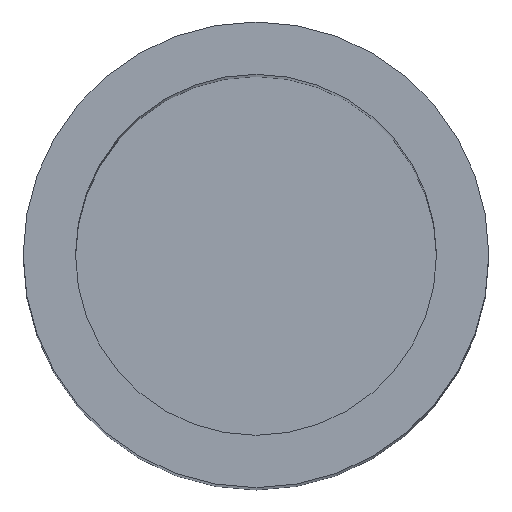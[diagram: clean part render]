
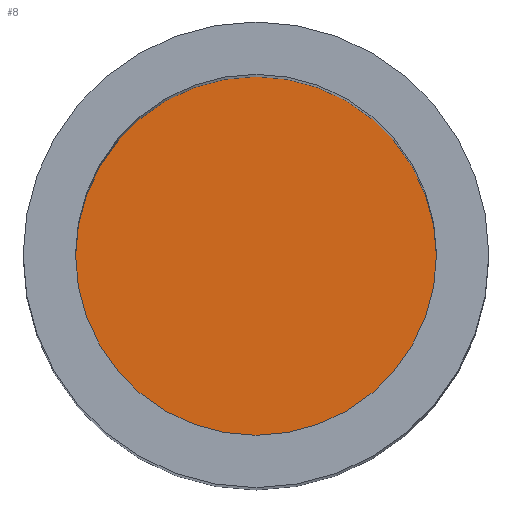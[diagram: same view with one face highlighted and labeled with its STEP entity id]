
A CAD part, top view. The second image highlights one B-rep face of the part: STEP entity #8.
In plain terms, the highlighted planar face has unit normal (0, 0, 1).
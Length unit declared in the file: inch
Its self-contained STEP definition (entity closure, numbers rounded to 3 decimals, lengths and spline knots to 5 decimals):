
#8 = ADVANCED_FACE ( 'NONE', ( #20 ), #34, .T. ) ;
#10 = VERTEX_POINT ( 'NONE', #22 ) ;
#14 = ORIENTED_EDGE ( 'NONE', *, *, #46, .T. ) ;
#20 = FACE_OUTER_BOUND ( 'NONE', #70, .T. ) ;
#22 = CARTESIAN_POINT ( 'NONE',  ( 0.5, 0., -7.615 ) ) ;
#34 = PLANE ( 'NONE',  #120 ) ;
#36 = DIRECTION ( 'NONE',  ( 0., 0., 1. ) ) ;
#41 = CARTESIAN_POINT ( 'NONE',  ( 0., 0., -7.615 ) ) ;
#46 = EDGE_CURVE ( 'NONE', #115, #10, #148, .T. ) ;
#54 = DIRECTION ( 'NONE',  ( -1., 0., 0. ) ) ;
#55 = DIRECTION ( 'NONE',  ( -1., 0., 0. ) ) ;
#60 = CARTESIAN_POINT ( 'NONE',  ( 0., 0., -7.615 ) ) ;
#68 = AXIS2_PLACEMENT_3D ( 'NONE', #104, #113, #108 ) ;
#70 = EDGE_LOOP ( 'NONE', ( #154, #14 ) ) ;
#81 = CARTESIAN_POINT ( 'NONE',  ( -0.5, 0., -7.615 ) ) ;
#104 = CARTESIAN_POINT ( 'NONE',  ( 0., 0., -7.615 ) ) ;
#108 = DIRECTION ( 'NONE',  ( -1., 0., 0. ) ) ;
#113 = DIRECTION ( 'NONE',  ( 0., 0., 1. ) ) ;
#115 = VERTEX_POINT ( 'NONE', #81 ) ;
#120 = AXIS2_PLACEMENT_3D ( 'NONE', #60, #122, #54 ) ;
#122 = DIRECTION ( 'NONE',  ( 0., 0., 1. ) ) ;
#148 = CIRCLE ( 'NONE', #68, 0.5 ) ;
#154 = ORIENTED_EDGE ( 'NONE', *, *, #217, .T. ) ;
#172 = AXIS2_PLACEMENT_3D ( 'NONE', #41, #36, #55 ) ;
#174 = CIRCLE ( 'NONE', #172, 0.5 ) ;
#217 = EDGE_CURVE ( 'NONE', #10, #115, #174, .T. ) ;
